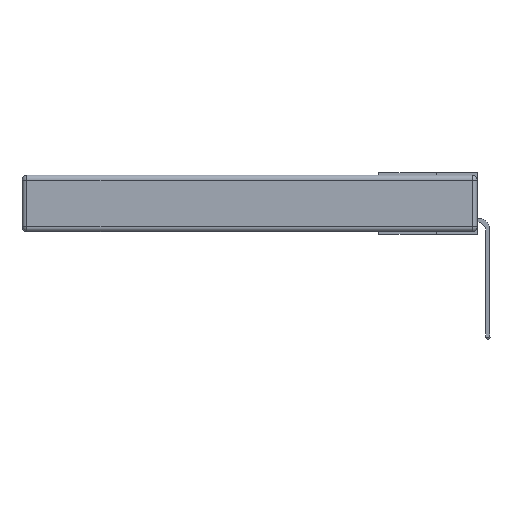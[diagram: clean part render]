
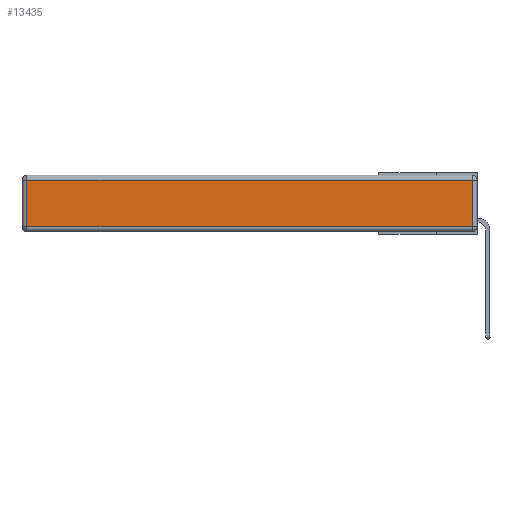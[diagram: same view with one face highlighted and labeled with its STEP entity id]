
A CAD part, left-side view. The second image highlights one B-rep face of the part: STEP entity #13435.
In plain terms, the highlighted planar face has unit normal (-1, 0, 0).
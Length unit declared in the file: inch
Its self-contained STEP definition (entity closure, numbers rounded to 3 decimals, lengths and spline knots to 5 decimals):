
#176 = CARTESIAN_POINT ( 'NONE',  ( 0., 2.72, -0.313 ) ) ;
#362 = LINE ( 'NONE', #10705, #10643 ) ;
#429 = VERTEX_POINT ( 'NONE', #176 ) ;
#447 = LINE ( 'NONE', #5026, #12936 ) ;
#487 = LINE ( 'NONE', #5625, #15051 ) ;
#491 = ORIENTED_EDGE ( 'NONE', *, *, #9216, .T. ) ;
#736 = VERTEX_POINT ( 'NONE', #8283 ) ;
#2076 = VECTOR ( 'NONE', #3894, 39.37008 ) ;
#2149 = DIRECTION ( 'NONE',  ( -1., 0., 0. ) ) ;
#2464 = LINE ( 'NONE', #11587, #2076 ) ;
#3402 = DIRECTION ( 'NONE',  ( 0., -1., 0. ) ) ;
#3793 = PLANE ( 'NONE',  #13569 ) ;
#3894 = DIRECTION ( 'NONE',  ( 0., 0., -1. ) ) ;
#4120 = FACE_OUTER_BOUND ( 'NONE', #12108, .T. ) ;
#4866 = DIRECTION ( 'NONE',  ( 0., 0., 1. ) ) ;
#5026 = CARTESIAN_POINT ( 'NONE',  ( 0., 2.75, -0.03 ) ) ;
#5126 = EDGE_CURVE ( 'NONE', #14344, #736, #447, .T. ) ;
#5625 = CARTESIAN_POINT ( 'NONE',  ( 0., 0.03, -0.343 ) ) ;
#8283 = CARTESIAN_POINT ( 'NONE',  ( 0., 2.72, -0.03 ) ) ;
#8760 = DIRECTION ( 'NONE',  ( 0., 1., 0. ) ) ;
#8865 = ORIENTED_EDGE ( 'NONE', *, *, #9457, .T. ) ;
#9216 = EDGE_CURVE ( 'NONE', #736, #429, #2464, .T. ) ;
#9457 = EDGE_CURVE ( 'NONE', #429, #14359, #362, .T. ) ;
#10122 = ORIENTED_EDGE ( 'NONE', *, *, #11388, .T. ) ;
#10643 = VECTOR ( 'NONE', #3402, 39.37008 ) ;
#10705 = CARTESIAN_POINT ( 'NONE',  ( 0., 0., -0.313 ) ) ;
#11056 = CARTESIAN_POINT ( 'NONE',  ( 0., 0.03, -0.03 ) ) ;
#11388 = EDGE_CURVE ( 'NONE', #14359, #14344, #487, .T. ) ;
#11573 = DIRECTION ( 'NONE',  ( 0., 0., 1. ) ) ;
#11587 = CARTESIAN_POINT ( 'NONE',  ( 0., 2.72, -0.343 ) ) ;
#12108 = EDGE_LOOP ( 'NONE', ( #8865, #10122, #12695, #491 ) ) ;
#12208 = CARTESIAN_POINT ( 'NONE',  ( 0., 0.03, -0.313 ) ) ;
#12289 = CARTESIAN_POINT ( 'NONE',  ( 0., 0., -0.343 ) ) ;
#12695 = ORIENTED_EDGE ( 'NONE', *, *, #5126, .T. ) ;
#12936 = VECTOR ( 'NONE', #8760, 39.37008 ) ;
#13435 = ADVANCED_FACE ( 'NONE', ( #4120 ), #3793, .T. ) ;
#13569 = AXIS2_PLACEMENT_3D ( 'NONE', #12289, #2149, #4866 ) ;
#14344 = VERTEX_POINT ( 'NONE', #11056 ) ;
#14359 = VERTEX_POINT ( 'NONE', #12208 ) ;
#15051 = VECTOR ( 'NONE', #11573, 39.37008 ) ;
